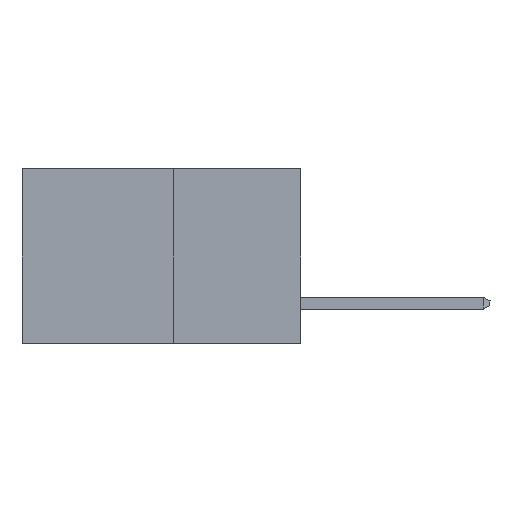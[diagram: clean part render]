
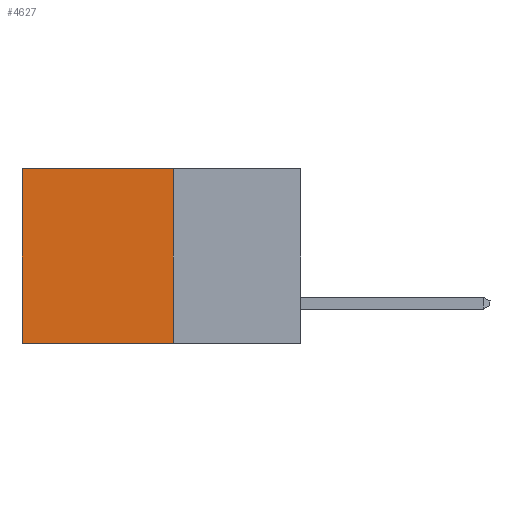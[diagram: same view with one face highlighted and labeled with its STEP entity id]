
A CAD part, left-side view. The second image highlights one B-rep face of the part: STEP entity #4627.
In plain terms, the highlighted planar face has unit normal (-1, 0, 0).
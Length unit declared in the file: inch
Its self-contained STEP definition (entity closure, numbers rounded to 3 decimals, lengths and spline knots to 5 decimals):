
#155 = ORIENTED_EDGE ( 'NONE', *, *, #3622, .T. ) ;
#532 = EDGE_CURVE ( 'NONE', #8363, #3995, #5296, .T. ) ;
#2315 = CARTESIAN_POINT ( 'NONE',  ( 0.277, 0.27, -0.37 ) ) ;
#3234 = CARTESIAN_POINT ( 'NONE',  ( 0.277, 0.27, -0.37 ) ) ;
#3310 = DIRECTION ( 'NONE',  ( 0., 0., -1. ) ) ;
#3622 = EDGE_CURVE ( 'NONE', #4274, #8363, #7570, .T. ) ;
#3995 = VERTEX_POINT ( 'NONE', #8594 ) ;
#4010 = ORIENTED_EDGE ( 'NONE', *, *, #532, .T. ) ;
#4258 = VECTOR ( 'NONE', #11041, 39.37008 ) ;
#4274 = VERTEX_POINT ( 'NONE', #6848 ) ;
#4627 = ADVANCED_FACE ( 'NONE', ( #7691 ), #4641, .F. ) ;
#4632 = DIRECTION ( 'NONE',  ( 0., 0., -1. ) ) ;
#4638 = DIRECTION ( 'NONE',  ( 1., 0., 0. ) ) ;
#4641 = PLANE ( 'NONE',  #7621 ) ;
#4727 = CARTESIAN_POINT ( 'NONE',  ( 0.277, 0.27, -0.37 ) ) ;
#5296 = LINE ( 'NONE', #12507, #12960 ) ;
#5490 = VECTOR ( 'NONE', #3310, 39.37008 ) ;
#5876 = EDGE_CURVE ( 'NONE', #12059, #3995, #6831, .T. ) ;
#6172 = EDGE_LOOP ( 'NONE', ( #4010, #6242, #6254, #155 ) ) ;
#6242 = ORIENTED_EDGE ( 'NONE', *, *, #5876, .F. ) ;
#6254 = ORIENTED_EDGE ( 'NONE', *, *, #10880, .F. ) ;
#6831 = LINE ( 'NONE', #8227, #12162 ) ;
#6848 = CARTESIAN_POINT ( 'NONE',  ( 0.277, 0.27, 0. ) ) ;
#7570 = LINE ( 'NONE', #11024, #4258 ) ;
#7621 = AXIS2_PLACEMENT_3D ( 'NONE', #4727, #4638, #4632 ) ;
#7691 = FACE_OUTER_BOUND ( 'NONE', #6172, .T. ) ;
#8167 = LINE ( 'NONE', #3234, #5490 ) ;
#8227 = CARTESIAN_POINT ( 'NONE',  ( 0.277, 0.27, -0.37 ) ) ;
#8363 = VERTEX_POINT ( 'NONE', #9032 ) ;
#8521 = DIRECTION ( 'NONE',  ( 0., 1., 0. ) ) ;
#8594 = CARTESIAN_POINT ( 'NONE',  ( 0.277, 0.59, -0.37 ) ) ;
#9032 = CARTESIAN_POINT ( 'NONE',  ( 0.277, 0.59, 0. ) ) ;
#10880 = EDGE_CURVE ( 'NONE', #4274, #12059, #8167, .T. ) ;
#11024 = CARTESIAN_POINT ( 'NONE',  ( 0.277, 0.27, 0. ) ) ;
#11041 = DIRECTION ( 'NONE',  ( 0., 1., 0. ) ) ;
#12059 = VERTEX_POINT ( 'NONE', #2315 ) ;
#12162 = VECTOR ( 'NONE', #8521, 39.37008 ) ;
#12326 = DIRECTION ( 'NONE',  ( 0., 0., -1. ) ) ;
#12507 = CARTESIAN_POINT ( 'NONE',  ( 0.277, 0.59, -0.37 ) ) ;
#12960 = VECTOR ( 'NONE', #12326, 39.37008 ) ;
